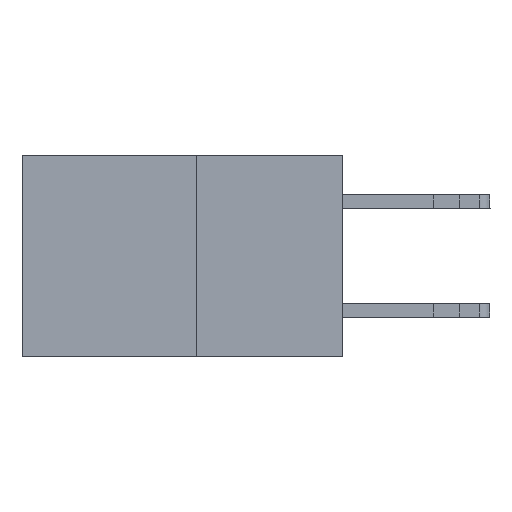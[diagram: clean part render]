
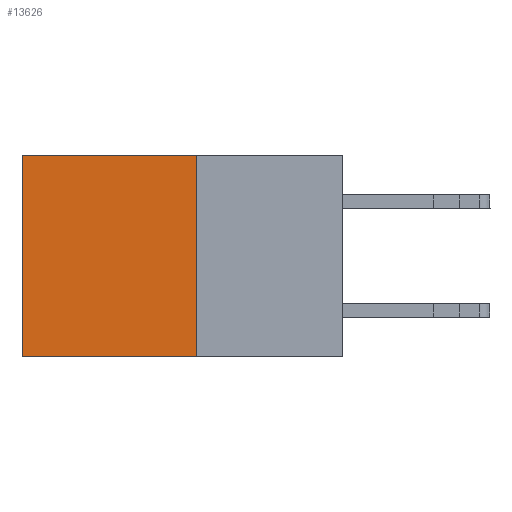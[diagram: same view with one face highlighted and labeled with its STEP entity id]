
A CAD part, left-side view. The second image highlights one B-rep face of the part: STEP entity #13626.
In plain terms, the highlighted planar face has unit normal (-1, 0, 0).
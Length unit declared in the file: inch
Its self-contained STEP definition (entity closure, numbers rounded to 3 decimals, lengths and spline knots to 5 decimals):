
#431 = EDGE_CURVE ( 'NONE', #15416, #15259, #12205, .T. ) ;
#1861 = LINE ( 'NONE', #10110, #12999 ) ;
#2579 = CARTESIAN_POINT ( 'NONE',  ( 0.277, 0.27, 0. ) ) ;
#3109 = FACE_OUTER_BOUND ( 'NONE', #17380, .T. ) ;
#3989 = PLANE ( 'NONE',  #13735 ) ;
#4364 = DIRECTION ( 'NONE',  ( 0., 0., -1. ) ) ;
#4411 = LINE ( 'NONE', #13930, #4855 ) ;
#4855 = VECTOR ( 'NONE', #6743, 39.37008 ) ;
#5447 = DIRECTION ( 'NONE',  ( 0., 0., -1. ) ) ;
#6441 = DIRECTION ( 'NONE',  ( 0., 1., 0. ) ) ;
#6743 = DIRECTION ( 'NONE',  ( 0., 0., -1. ) ) ;
#6792 = VERTEX_POINT ( 'NONE', #11282 ) ;
#7339 = EDGE_CURVE ( 'NONE', #15259, #6792, #4411, .T. ) ;
#7927 = VECTOR ( 'NONE', #6441, 39.37008 ) ;
#8411 = CARTESIAN_POINT ( 'NONE',  ( 0.277, 0.27, -0.37 ) ) ;
#9388 = ORIENTED_EDGE ( 'NONE', *, *, #7339, .T. ) ;
#9431 = ORIENTED_EDGE ( 'NONE', *, *, #9914, .F. ) ;
#9557 = ORIENTED_EDGE ( 'NONE', *, *, #11760, .F. ) ;
#9587 = ORIENTED_EDGE ( 'NONE', *, *, #431, .T. ) ;
#9674 = CARTESIAN_POINT ( 'NONE',  ( 0.277, 0.27, 0. ) ) ;
#9914 = EDGE_CURVE ( 'NONE', #13719, #6792, #1861, .T. ) ;
#10110 = CARTESIAN_POINT ( 'NONE',  ( 0.277, 0.27, -0.37 ) ) ;
#10244 = CARTESIAN_POINT ( 'NONE',  ( 0.277, 0.27, -0.37 ) ) ;
#11282 = CARTESIAN_POINT ( 'NONE',  ( 0.277, 0.59, -0.37 ) ) ;
#11538 = CARTESIAN_POINT ( 'NONE',  ( 0.277, 0.27, -0.37 ) ) ;
#11760 = EDGE_CURVE ( 'NONE', #15416, #13719, #16108, .T. ) ;
#12205 = LINE ( 'NONE', #9674, #7927 ) ;
#12287 = VECTOR ( 'NONE', #4364, 39.37008 ) ;
#12999 = VECTOR ( 'NONE', #18565, 39.37008 ) ;
#13626 = ADVANCED_FACE ( 'NONE', ( #3109 ), #3989, .F. ) ;
#13719 = VERTEX_POINT ( 'NONE', #11538 ) ;
#13735 = AXIS2_PLACEMENT_3D ( 'NONE', #8411, #14151, #5447 ) ;
#13930 = CARTESIAN_POINT ( 'NONE',  ( 0.277, 0.59, -0.37 ) ) ;
#14151 = DIRECTION ( 'NONE',  ( 1., 0., 0. ) ) ;
#15259 = VERTEX_POINT ( 'NONE', #15321 ) ;
#15321 = CARTESIAN_POINT ( 'NONE',  ( 0.277, 0.59, 0. ) ) ;
#15416 = VERTEX_POINT ( 'NONE', #2579 ) ;
#16108 = LINE ( 'NONE', #10244, #12287 ) ;
#17380 = EDGE_LOOP ( 'NONE', ( #9388, #9431, #9557, #9587 ) ) ;
#18565 = DIRECTION ( 'NONE',  ( 0., 1., 0. ) ) ;
